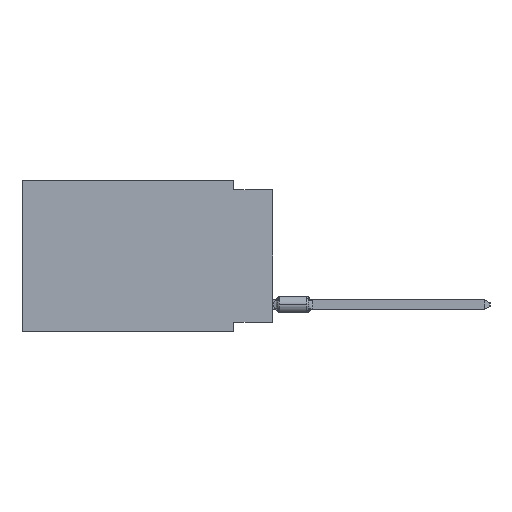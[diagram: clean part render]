
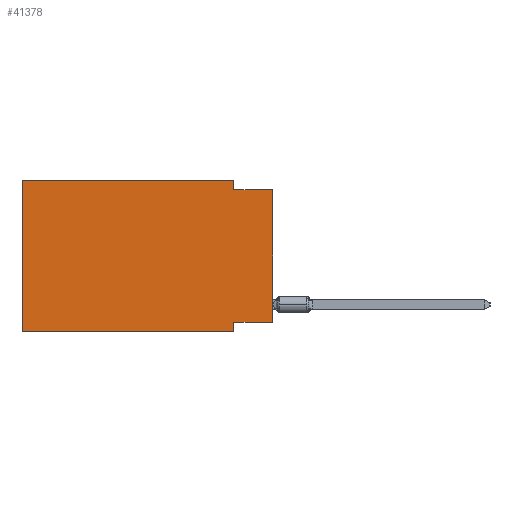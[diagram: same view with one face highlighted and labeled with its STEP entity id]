
A CAD part, left-side view. The second image highlights one B-rep face of the part: STEP entity #41378.
In plain terms, the highlighted planar face has unit normal (-1, 0, 0).
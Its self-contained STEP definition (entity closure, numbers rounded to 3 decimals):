
#527 = CARTESIAN_POINT ( 'NONE',  ( 0., 2.54, 0. ) ) ;
#582 = ORIENTED_EDGE ( 'NONE', *, *, #59305, .T. ) ;
#1116 = VERTEX_POINT ( 'NONE', #12076 ) ;
#1318 = EDGE_CURVE ( 'NONE', #10405, #1880, #47607, .T. ) ;
#1880 = VERTEX_POINT ( 'NONE', #14488 ) ;
#2590 = EDGE_CURVE ( 'NONE', #10405, #5652, #36998, .T. ) ;
#3051 = DIRECTION ( 'NONE',  ( 1., 0., 0. ) ) ;
#3283 = VECTOR ( 'NONE', #16346, 1000. ) ;
#5576 = CARTESIAN_POINT ( 'NONE',  ( 0., 0., 0. ) ) ;
#5652 = VERTEX_POINT ( 'NONE', #38622 ) ;
#8523 = DIRECTION ( 'NONE',  ( 0., 0., 1. ) ) ;
#10405 = VERTEX_POINT ( 'NONE', #16555 ) ;
#10453 = LINE ( 'NONE', #29177, #11925 ) ;
#11090 = VERTEX_POINT ( 'NONE', #527 ) ;
#11506 = VECTOR ( 'NONE', #8523, 1000. ) ;
#11717 = EDGE_CURVE ( 'NONE', #34108, #1880, #29930, .T. ) ;
#11925 = VECTOR ( 'NONE', #24878, 1000. ) ;
#12076 = CARTESIAN_POINT ( 'NONE',  ( 0., 2.54, -9.906 ) ) ;
#12721 = VECTOR ( 'NONE', #15571, 1000. ) ;
#13066 = DIRECTION ( 'NONE',  ( 0., 1., 0. ) ) ;
#13133 = LINE ( 'NONE', #50553, #11506 ) ;
#14396 = AXIS2_PLACEMENT_3D ( 'NONE', #47964, #3051, #33874 ) ;
#14488 = CARTESIAN_POINT ( 'NONE',  ( 0., 0., -0.635 ) ) ;
#15010 = ORIENTED_EDGE ( 'NONE', *, *, #2590, .F. ) ;
#15571 = DIRECTION ( 'NONE',  ( 0., 0., -1. ) ) ;
#16297 = ORIENTED_EDGE ( 'NONE', *, *, #1318, .T. ) ;
#16346 = DIRECTION ( 'NONE',  ( 0., -1., 0. ) ) ;
#16555 = CARTESIAN_POINT ( 'NONE',  ( 0., 0., -9.271 ) ) ;
#20735 = VERTEX_POINT ( 'NONE', #50554 ) ;
#22912 = ORIENTED_EDGE ( 'NONE', *, *, #42725, .F. ) ;
#24304 = DIRECTION ( 'NONE',  ( 0., 0., 1. ) ) ;
#24776 = CARTESIAN_POINT ( 'NONE',  ( 0., 2.54, -9.906 ) ) ;
#24878 = DIRECTION ( 'NONE',  ( 0., -1., 0. ) ) ;
#25129 = ORIENTED_EDGE ( 'NONE', *, *, #56948, .F. ) ;
#25979 = DIRECTION ( 'NONE',  ( 0., 0., -1. ) ) ;
#26663 = ORIENTED_EDGE ( 'NONE', *, *, #56944, .F. ) ;
#29177 = CARTESIAN_POINT ( 'NONE',  ( 0., 16.383, -9.906 ) ) ;
#29930 = LINE ( 'NONE', #39729, #39642 ) ;
#32363 = CARTESIAN_POINT ( 'NONE',  ( 0., 2.54, -0.635 ) ) ;
#32396 = CARTESIAN_POINT ( 'NONE',  ( 0., 0., -9.271 ) ) ;
#33874 = DIRECTION ( 'NONE',  ( 0., 0., -1. ) ) ;
#34108 = VERTEX_POINT ( 'NONE', #32363 ) ;
#36998 = LINE ( 'NONE', #32396, #50523 ) ;
#37373 = VERTEX_POINT ( 'NONE', #56257 ) ;
#38622 = CARTESIAN_POINT ( 'NONE',  ( 0., 2.54, -9.271 ) ) ;
#39163 = VECTOR ( 'NONE', #25979, 1000. ) ;
#39642 = VECTOR ( 'NONE', #59057, 1000. ) ;
#39729 = CARTESIAN_POINT ( 'NONE',  ( 0., 0., -0.635 ) ) ;
#41378 = ADVANCED_FACE ( 'NONE', ( #53164 ), #48254, .F. ) ;
#42725 = EDGE_CURVE ( 'NONE', #20735, #37373, #13133, .T. ) ;
#43771 = ORIENTED_EDGE ( 'NONE', *, *, #11717, .F. ) ;
#44576 = LINE ( 'NONE', #58379, #3283 ) ;
#47607 = LINE ( 'NONE', #5576, #60220 ) ;
#47964 = CARTESIAN_POINT ( 'NONE',  ( 0., 16.383, 0. ) ) ;
#48254 = PLANE ( 'NONE',  #14396 ) ;
#49305 = EDGE_CURVE ( 'NONE', #37373, #11090, #44576, .T. ) ;
#50523 = VECTOR ( 'NONE', #13066, 1000. ) ;
#50553 = CARTESIAN_POINT ( 'NONE',  ( 0., 16.383, 0. ) ) ;
#50554 = CARTESIAN_POINT ( 'NONE',  ( 0., 16.383, -9.906 ) ) ;
#52992 = CARTESIAN_POINT ( 'NONE',  ( 0., 2.54, 0. ) ) ;
#53164 = FACE_OUTER_BOUND ( 'NONE', #54426, .T. ) ;
#53287 = LINE ( 'NONE', #52992, #12721 ) ;
#54426 = EDGE_LOOP ( 'NONE', ( #16297, #43771, #25129, #60412, #22912, #582, #26663, #15010 ) ) ;
#56257 = CARTESIAN_POINT ( 'NONE',  ( 0., 16.383, 0. ) ) ;
#56944 = EDGE_CURVE ( 'NONE', #5652, #1116, #57599, .T. ) ;
#56948 = EDGE_CURVE ( 'NONE', #11090, #34108, #53287, .T. ) ;
#57599 = LINE ( 'NONE', #24776, #39163 ) ;
#58379 = CARTESIAN_POINT ( 'NONE',  ( 0., 16.383, 0. ) ) ;
#59057 = DIRECTION ( 'NONE',  ( 0., -1., 0. ) ) ;
#59305 = EDGE_CURVE ( 'NONE', #20735, #1116, #10453, .T. ) ;
#60220 = VECTOR ( 'NONE', #24304, 1000. ) ;
#60412 = ORIENTED_EDGE ( 'NONE', *, *, #49305, .F. ) ;
